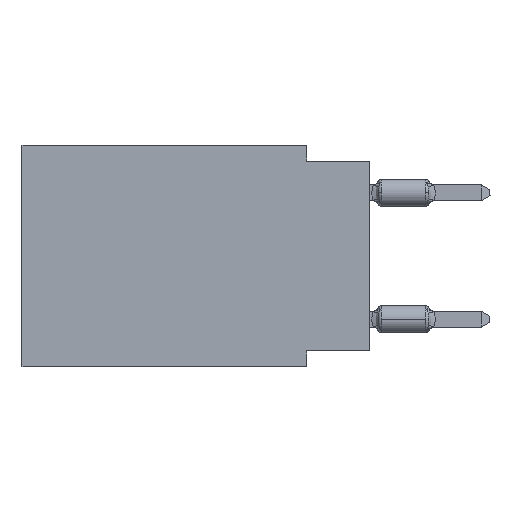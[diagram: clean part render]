
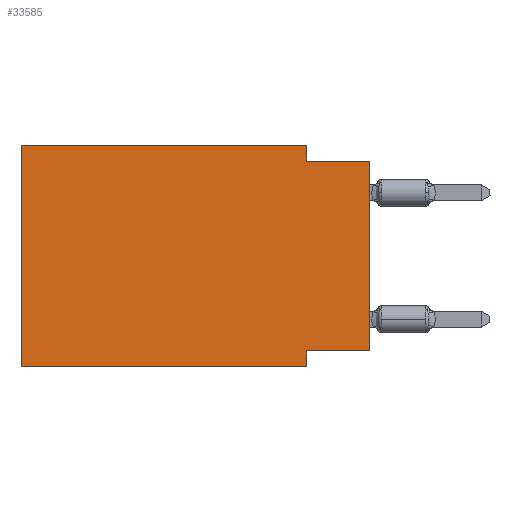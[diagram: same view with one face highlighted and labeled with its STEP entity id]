
A CAD part, left-side view. The second image highlights one B-rep face of the part: STEP entity #33585.
In plain terms, the highlighted planar face has unit normal (-1, 0, 0).
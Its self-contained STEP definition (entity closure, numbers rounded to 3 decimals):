
#97 = DIRECTION ( 'NONE',  ( 0., 0., 1. ) ) ;
#241 = DIRECTION ( 'NONE',  ( 0., -1., 0. ) ) ;
#550 = CARTESIAN_POINT ( 'NONE',  ( 0., 13.97, 0. ) ) ;
#832 = VECTOR ( 'NONE', #97, 1000. ) ;
#1158 = ORIENTED_EDGE ( 'NONE', *, *, #2674, .F. ) ;
#1826 = ORIENTED_EDGE ( 'NONE', *, *, #32285, .T. ) ;
#2428 = VECTOR ( 'NONE', #25212, 1000. ) ;
#2674 = EDGE_CURVE ( 'NONE', #31570, #7331, #28570, .T. ) ;
#3215 = LINE ( 'NONE', #33995, #27175 ) ;
#4272 = LINE ( 'NONE', #15962, #2428 ) ;
#4441 = VERTEX_POINT ( 'NONE', #38753 ) ;
#7237 = EDGE_LOOP ( 'NONE', ( #1826, #8371, #17371, #1158, #20389, #8733, #36819, #36405 ) ) ;
#7331 = VERTEX_POINT ( 'NONE', #34597 ) ;
#7504 = LINE ( 'NONE', #8101, #8469 ) ;
#7671 = EDGE_CURVE ( 'NONE', #4441, #31194, #11256, .T. ) ;
#8101 = CARTESIAN_POINT ( 'NONE',  ( 0., 2.54, 0. ) ) ;
#8371 = ORIENTED_EDGE ( 'NONE', *, *, #29007, .F. ) ;
#8469 = VECTOR ( 'NONE', #20400, 1000. ) ;
#8471 = LINE ( 'NONE', #20761, #12191 ) ;
#8700 = CARTESIAN_POINT ( 'NONE',  ( 0., 2.54, -8.89 ) ) ;
#8733 = ORIENTED_EDGE ( 'NONE', *, *, #19956, .T. ) ;
#9552 = LINE ( 'NONE', #37293, #832 ) ;
#9670 = CARTESIAN_POINT ( 'NONE',  ( 0., 13.97, 0. ) ) ;
#10240 = VERTEX_POINT ( 'NONE', #18480 ) ;
#10246 = CARTESIAN_POINT ( 'NONE',  ( 0., 13.97, -8.89 ) ) ;
#11256 = LINE ( 'NONE', #26952, #39036 ) ;
#11778 = CARTESIAN_POINT ( 'NONE',  ( 0., 13.97, 0. ) ) ;
#12191 = VECTOR ( 'NONE', #33013, 1000. ) ;
#12369 = DIRECTION ( 'NONE',  ( 0., 0., -1. ) ) ;
#14366 = VECTOR ( 'NONE', #19338, 1000. ) ;
#15403 = FACE_OUTER_BOUND ( 'NONE', #7237, .T. ) ;
#15962 = CARTESIAN_POINT ( 'NONE',  ( 0., 2.54, -8.89 ) ) ;
#17371 = ORIENTED_EDGE ( 'NONE', *, *, #19680, .F. ) ;
#17692 = DIRECTION ( 'NONE',  ( 0., 1., 0. ) ) ;
#18480 = CARTESIAN_POINT ( 'NONE',  ( 0., 2.54, -0.635 ) ) ;
#18771 = VECTOR ( 'NONE', #241, 1000. ) ;
#19338 = DIRECTION ( 'NONE',  ( 0., -1., 0. ) ) ;
#19680 = EDGE_CURVE ( 'NONE', #7331, #10240, #7504, .T. ) ;
#19831 = VERTEX_POINT ( 'NONE', #8700 ) ;
#19956 = EDGE_CURVE ( 'NONE', #20491, #19831, #31212, .T. ) ;
#20389 = ORIENTED_EDGE ( 'NONE', *, *, #32013, .F. ) ;
#20400 = DIRECTION ( 'NONE',  ( 0., 0., -1. ) ) ;
#20491 = VERTEX_POINT ( 'NONE', #10246 ) ;
#20761 = CARTESIAN_POINT ( 'NONE',  ( 0., 0., -0.635 ) ) ;
#21058 = PLANE ( 'NONE',  #32299 ) ;
#23905 = VERTEX_POINT ( 'NONE', #34010 ) ;
#25212 = DIRECTION ( 'NONE',  ( 0., 0., -1. ) ) ;
#26952 = CARTESIAN_POINT ( 'NONE',  ( 0., 0., -8.255 ) ) ;
#27175 = VECTOR ( 'NONE', #33198, 1000. ) ;
#28212 = CARTESIAN_POINT ( 'NONE',  ( 0., 13.97, -8.89 ) ) ;
#28570 = LINE ( 'NONE', #9670, #14366 ) ;
#29007 = EDGE_CURVE ( 'NONE', #10240, #23905, #8471, .T. ) ;
#31169 = CARTESIAN_POINT ( 'NONE',  ( 0., 2.54, -8.255 ) ) ;
#31194 = VERTEX_POINT ( 'NONE', #31169 ) ;
#31212 = LINE ( 'NONE', #28212, #18771 ) ;
#31570 = VERTEX_POINT ( 'NONE', #550 ) ;
#32013 = EDGE_CURVE ( 'NONE', #20491, #31570, #9552, .T. ) ;
#32285 = EDGE_CURVE ( 'NONE', #4441, #23905, #3215, .T. ) ;
#32299 = AXIS2_PLACEMENT_3D ( 'NONE', #11778, #33900, #12369 ) ;
#33013 = DIRECTION ( 'NONE',  ( 0., -1., 0. ) ) ;
#33198 = DIRECTION ( 'NONE',  ( 0., 0., 1. ) ) ;
#33585 = ADVANCED_FACE ( 'NONE', ( #15403 ), #21058, .F. ) ;
#33900 = DIRECTION ( 'NONE',  ( 1., 0., 0. ) ) ;
#33995 = CARTESIAN_POINT ( 'NONE',  ( 0., 0., 0. ) ) ;
#34010 = CARTESIAN_POINT ( 'NONE',  ( 0., 0., -0.635 ) ) ;
#34597 = CARTESIAN_POINT ( 'NONE',  ( 0., 2.54, 0. ) ) ;
#36405 = ORIENTED_EDGE ( 'NONE', *, *, #7671, .F. ) ;
#36680 = EDGE_CURVE ( 'NONE', #31194, #19831, #4272, .T. ) ;
#36819 = ORIENTED_EDGE ( 'NONE', *, *, #36680, .F. ) ;
#37293 = CARTESIAN_POINT ( 'NONE',  ( 0., 13.97, 0. ) ) ;
#38753 = CARTESIAN_POINT ( 'NONE',  ( 0., 0., -8.255 ) ) ;
#39036 = VECTOR ( 'NONE', #17692, 1000. ) ;
